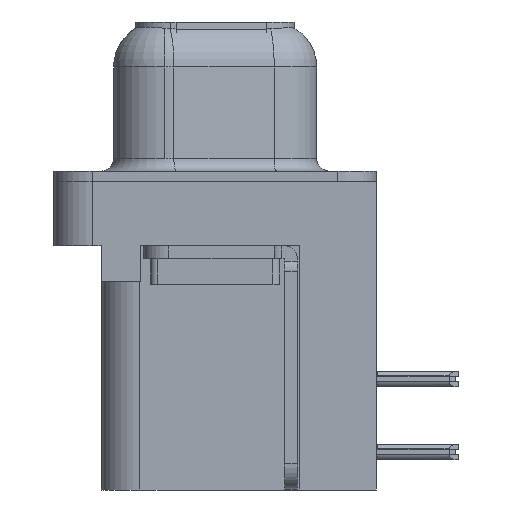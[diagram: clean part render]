
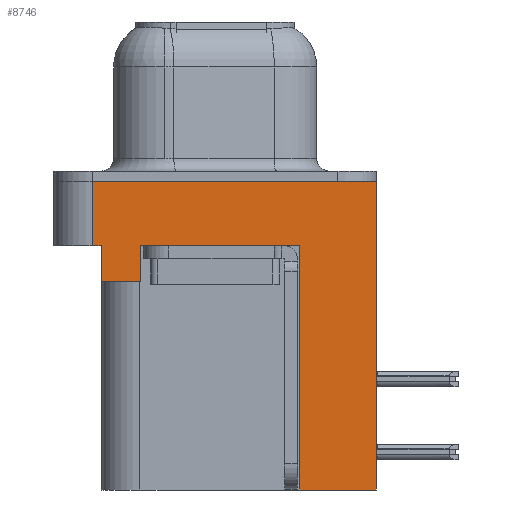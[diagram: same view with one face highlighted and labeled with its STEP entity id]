
A CAD part, left-side view. The second image highlights one B-rep face of the part: STEP entity #8746.
In plain terms, the highlighted planar face has unit normal (-1, 0, 0).
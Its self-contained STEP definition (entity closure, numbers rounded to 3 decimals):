
#609 = VERTEX_POINT ( 'NONE', #18560 ) ;
#761 = EDGE_CURVE ( 'NONE', #26934, #14360, #19569, .T. ) ;
#913 = CARTESIAN_POINT ( 'NONE',  ( -3., -3.295, -12. ) ) ;
#1186 = CARTESIAN_POINT ( 'NONE',  ( -3., -6.275, -2.5 ) ) ;
#1719 = EDGE_CURVE ( 'NONE', #609, #9648, #27158, .T. ) ;
#1965 = ORIENTED_EDGE ( 'NONE', *, *, #14845, .T. ) ;
#2225 = DIRECTION ( 'NONE',  ( 0., 0., 1. ) ) ;
#2446 = EDGE_CURVE ( 'NONE', #23923, #14360, #6031, .T. ) ;
#2500 = LINE ( 'NONE', #28057, #7704 ) ;
#3166 = FACE_OUTER_BOUND ( 'NONE', #28555, .T. ) ;
#3355 = EDGE_CURVE ( 'NONE', #26618, #9648, #25334, .T. ) ;
#4461 = PLANE ( 'NONE',  #27585 ) ;
#5221 = VECTOR ( 'NONE', #7910, 1000. ) ;
#5327 = ORIENTED_EDGE ( 'NONE', *, *, #7897, .T. ) ;
#5598 = VERTEX_POINT ( 'NONE', #9386 ) ;
#6031 = LINE ( 'NONE', #14392, #12671 ) ;
#6963 = ORIENTED_EDGE ( 'NONE', *, *, #28402, .F. ) ;
#7704 = VECTOR ( 'NONE', #19355, 1000. ) ;
#7895 = DIRECTION ( 'NONE',  ( 0., -1., 0. ) ) ;
#7897 = EDGE_CURVE ( 'NONE', #5598, #15672, #2500, .T. ) ;
#7910 = DIRECTION ( 'NONE',  ( 0., 0., 1. ) ) ;
#8746 = ADVANCED_FACE ( 'NONE', ( #3166 ), #4461, .T. ) ;
#9125 = EDGE_CURVE ( 'NONE', #9405, #26618, #20065, .T. ) ;
#9381 = CARTESIAN_POINT ( 'NONE',  ( -3., -3.295, -2.5 ) ) ;
#9386 = CARTESIAN_POINT ( 'NONE',  ( -3., -6.275, -12. ) ) ;
#9405 = VERTEX_POINT ( 'NONE', #9692 ) ;
#9605 = LINE ( 'NONE', #913, #20675 ) ;
#9648 = VERTEX_POINT ( 'NONE', #11624 ) ;
#9692 = CARTESIAN_POINT ( 'NONE',  ( -3., 2.895, -3.9 ) ) ;
#10049 = DIRECTION ( 'NONE',  ( 0., -1., 0. ) ) ;
#10840 = ORIENTED_EDGE ( 'NONE', *, *, #3355, .F. ) ;
#11624 = CARTESIAN_POINT ( 'NONE',  ( -3., 4.425, -2.5 ) ) ;
#12671 = VECTOR ( 'NONE', #20847, 1000. ) ;
#12810 = DIRECTION ( 'NONE',  ( 0., 1., 0. ) ) ;
#13378 = VECTOR ( 'NONE', #14976, 1000. ) ;
#13587 = ORIENTED_EDGE ( 'NONE', *, *, #1719, .T. ) ;
#14260 = VECTOR ( 'NONE', #20132, 1000. ) ;
#14360 = VERTEX_POINT ( 'NONE', #9381 ) ;
#14392 = CARTESIAN_POINT ( 'NONE',  ( -3., -3.295, -12. ) ) ;
#14430 = CARTESIAN_POINT ( 'NONE',  ( -3., -3.295, -12. ) ) ;
#14845 = EDGE_CURVE ( 'NONE', #9405, #26934, #26326, .T. ) ;
#14976 = DIRECTION ( 'NONE',  ( 0., -1., 0. ) ) ;
#15428 = ORIENTED_EDGE ( 'NONE', *, *, #2446, .F. ) ;
#15672 = VERTEX_POINT ( 'NONE', #16559 ) ;
#15707 = CARTESIAN_POINT ( 'NONE',  ( -3., 4.425, -3.9 ) ) ;
#15850 = EDGE_CURVE ( 'NONE', #28009, #15672, #24092, .T. ) ;
#16559 = CARTESIAN_POINT ( 'NONE',  ( -3., -6.275, 0. ) ) ;
#16575 = CARTESIAN_POINT ( 'NONE',  ( -3., 2.895, -2.5 ) ) ;
#16817 = VECTOR ( 'NONE', #10049, 1000. ) ;
#16974 = CARTESIAN_POINT ( 'NONE',  ( -3., -6.275, -2.5 ) ) ;
#17524 = CARTESIAN_POINT ( 'NONE',  ( -3., 4.775, 0. ) ) ;
#17706 = DIRECTION ( 'NONE',  ( -1., 0., 0. ) ) ;
#18411 = ORIENTED_EDGE ( 'NONE', *, *, #27563, .F. ) ;
#18560 = CARTESIAN_POINT ( 'NONE',  ( -3., 4.775, -2.5 ) ) ;
#19252 = VECTOR ( 'NONE', #7895, 1000. ) ;
#19355 = DIRECTION ( 'NONE',  ( 0., 0., 1. ) ) ;
#19451 = VECTOR ( 'NONE', #2225, 1000. ) ;
#19560 = ORIENTED_EDGE ( 'NONE', *, *, #761, .T. ) ;
#19569 = LINE ( 'NONE', #1186, #19252 ) ;
#19576 = DIRECTION ( 'NONE',  ( 0., 0., 1. ) ) ;
#19817 = DIRECTION ( 'NONE',  ( 0., 0., 1. ) ) ;
#20065 = LINE ( 'NONE', #15707, #14260 ) ;
#20132 = DIRECTION ( 'NONE',  ( 0., 1., 0. ) ) ;
#20523 = CARTESIAN_POINT ( 'NONE',  ( -3., 4.425, -3.9 ) ) ;
#20675 = VECTOR ( 'NONE', #12810, 1000. ) ;
#20747 = ORIENTED_EDGE ( 'NONE', *, *, #15850, .F. ) ;
#20847 = DIRECTION ( 'NONE',  ( 0., 0., 1. ) ) ;
#21145 = CARTESIAN_POINT ( 'NONE',  ( -3., 2.895, -3.9 ) ) ;
#22092 = VECTOR ( 'NONE', #19576, 1000. ) ;
#23923 = VERTEX_POINT ( 'NONE', #14430 ) ;
#24036 = CARTESIAN_POINT ( 'NONE',  ( -3., 4.775, -2.5 ) ) ;
#24086 = CARTESIAN_POINT ( 'NONE',  ( -3., -6.275, -2.5 ) ) ;
#24092 = LINE ( 'NONE', #25297, #16817 ) ;
#25297 = CARTESIAN_POINT ( 'NONE',  ( -3., -6.275, 0. ) ) ;
#25334 = LINE ( 'NONE', #26685, #19451 ) ;
#25436 = ORIENTED_EDGE ( 'NONE', *, *, #9125, .F. ) ;
#25565 = LINE ( 'NONE', #24036, #22092 ) ;
#26326 = LINE ( 'NONE', #21145, #5221 ) ;
#26618 = VERTEX_POINT ( 'NONE', #20523 ) ;
#26685 = CARTESIAN_POINT ( 'NONE',  ( -3., 4.425, -3.9 ) ) ;
#26934 = VERTEX_POINT ( 'NONE', #16575 ) ;
#27158 = LINE ( 'NONE', #16974, #13378 ) ;
#27563 = EDGE_CURVE ( 'NONE', #609, #28009, #25565, .T. ) ;
#27585 = AXIS2_PLACEMENT_3D ( 'NONE', #24086, #17706, #19817 ) ;
#28009 = VERTEX_POINT ( 'NONE', #17524 ) ;
#28057 = CARTESIAN_POINT ( 'NONE',  ( -3., -6.275, -2.5 ) ) ;
#28402 = EDGE_CURVE ( 'NONE', #5598, #23923, #9605, .T. ) ;
#28555 = EDGE_LOOP ( 'NONE', ( #20747, #18411, #13587, #10840, #25436, #1965, #19560, #15428, #6963, #5327 ) ) ;
